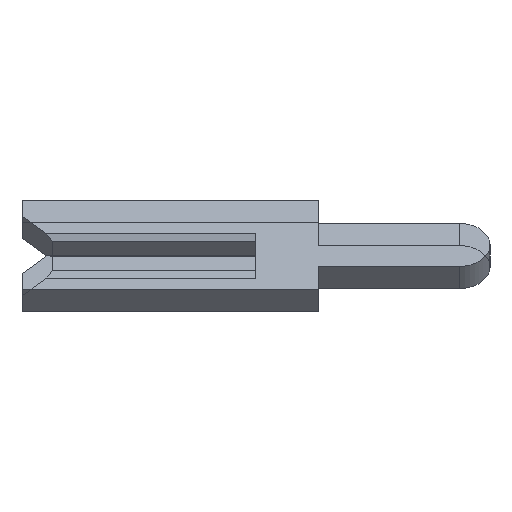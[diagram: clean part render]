
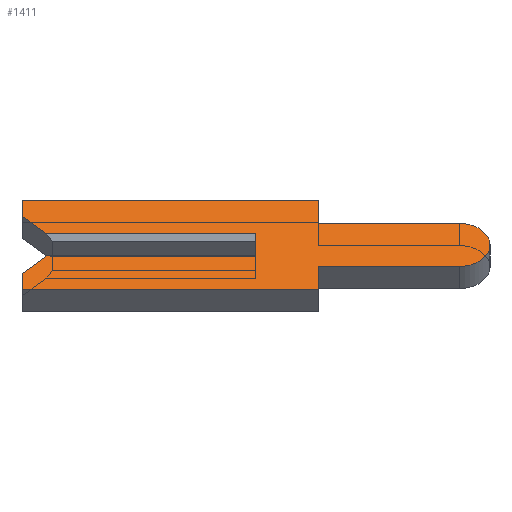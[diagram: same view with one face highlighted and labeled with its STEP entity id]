
A CAD part, left-side view. The second image highlights one B-rep face of the part: STEP entity #1411.
In plain terms, the highlighted face is planar.
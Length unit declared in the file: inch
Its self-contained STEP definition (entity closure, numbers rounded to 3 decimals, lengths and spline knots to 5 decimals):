
#4 = DIRECTION ( 'NONE',  ( 0., 0., 1. ) ) ;
#63 = VECTOR ( 'NONE', #1953, 39.37008 ) ;
#79 = VERTEX_POINT ( 'NONE', #1775 ) ;
#87 = EDGE_CURVE ( 'NONE', #1081, #1025, #403, .T. ) ;
#110 = VECTOR ( 'NONE', #1761, 39.37008 ) ;
#135 = VECTOR ( 'NONE', #1504, 39.37008 ) ;
#187 = CARTESIAN_POINT ( 'NONE',  ( -0.01, 0.1305, -0.0065 ) ) ;
#204 = VERTEX_POINT ( 'NONE', #2115 ) ;
#206 = AXIS2_PLACEMENT_3D ( 'NONE', #1594, #223, #1454 ) ;
#212 = ORIENTED_EDGE ( 'NONE', *, *, #1469, .F. ) ;
#223 = DIRECTION ( 'NONE',  ( 1., 0., 0. ) ) ;
#286 = VERTEX_POINT ( 'NONE', #1499 ) ;
#288 = CARTESIAN_POINT ( 'NONE',  ( -0.01, -0.1305, -0.01 ) ) ;
#289 = LINE ( 'NONE', #288, #135 ) ;
#359 = PLANE ( 'NONE',  #206 ) ;
#361 = VERTEX_POINT ( 'NONE', #1826 ) ;
#364 = CARTESIAN_POINT ( 'NONE',  ( -0.01, 0.15, 0.01 ) ) ;
#365 = VERTEX_POINT ( 'NONE', #1346 ) ;
#384 = CARTESIAN_POINT ( 'NONE',  ( -0.01, 0.15, 0.04 ) ) ;
#403 = LINE ( 'NONE', #755, #1865 ) ;
#416 = CARTESIAN_POINT ( 'NONE',  ( -0.01, 0.15, 0.04 ) ) ;
#417 = VERTEX_POINT ( 'NONE', #461 ) ;
#424 = LINE ( 'NONE', #416, #2146 ) ;
#461 = CARTESIAN_POINT ( 'NONE',  ( -0.01, 0.15, 0.026 ) ) ;
#474 = ORIENTED_EDGE ( 'NONE', *, *, #1277, .F. ) ;
#499 = CARTESIAN_POINT ( 'NONE',  ( -0.01, -0.04, 0.0195 ) ) ;
#509 = VECTOR ( 'NONE', #787, 39.37008 ) ;
#512 = LINE ( 'NONE', #1619, #63 ) ;
#513 = EDGE_CURVE ( 'NONE', #286, #204, #289, .T. ) ;
#547 = EDGE_CURVE ( 'NONE', #1768, #417, #993, .T. ) ;
#562 = CARTESIAN_POINT ( 'NONE',  ( -0.01, -0.04, -0.0195 ) ) ;
#570 = ORIENTED_EDGE ( 'NONE', *, *, #87, .F. ) ;
#598 = CIRCLE ( 'NONE', #1952, 0.0195 ) ;
#602 = CARTESIAN_POINT ( 'NONE',  ( -0.01, -0.04, -0.0195 ) ) ;
#607 = DIRECTION ( 'NONE',  ( 1., 0., 0. ) ) ;
#616 = LINE ( 'NONE', #1296, #2098 ) ;
#618 = DIRECTION ( 'NONE',  ( 0., 0., 1. ) ) ;
#634 = ORIENTED_EDGE ( 'NONE', *, *, #693, .F. ) ;
#638 = CARTESIAN_POINT ( 'NONE',  ( -0.01, 0.1305, 0.0065 ) ) ;
#642 = FACE_OUTER_BOUND ( 'NONE', #882, .T. ) ;
#693 = EDGE_CURVE ( 'NONE', #417, #1268, #828, .T. ) ;
#722 = LINE ( 'NONE', #187, #110 ) ;
#754 = VECTOR ( 'NONE', #1513, 39.37008 ) ;
#755 = CARTESIAN_POINT ( 'NONE',  ( -0.01, -0.04, 0.0195 ) ) ;
#776 = ORIENTED_EDGE ( 'NONE', *, *, #1968, .F. ) ;
#787 = DIRECTION ( 'NONE',  ( 0., 0., 1. ) ) ;
#802 = VECTOR ( 'NONE', #4, 39.37008 ) ;
#828 = LINE ( 'NONE', #865, #802 ) ;
#865 = CARTESIAN_POINT ( 'NONE',  ( -0.01, 0.15, 0.026 ) ) ;
#876 = VERTEX_POINT ( 'NONE', #1007 ) ;
#882 = EDGE_LOOP ( 'NONE', ( #1043, #474, #931, #1892, #2071, #776, #1511, #1441, #1754, #570, #212, #1570, #634, #1565 ) ) ;
#921 = DIRECTION ( 'NONE',  ( 0., -1., 0. ) ) ;
#931 = ORIENTED_EDGE ( 'NONE', *, *, #513, .F. ) ;
#944 = DIRECTION ( 'NONE',  ( 0., 1., 0. ) ) ;
#962 = LINE ( 'NONE', #562, #1835 ) ;
#993 = LINE ( 'NONE', #638, #754 ) ;
#1007 = CARTESIAN_POINT ( 'NONE',  ( -0.01, 0.15, -0.04 ) ) ;
#1024 = LINE ( 'NONE', #364, #1440 ) ;
#1025 = VERTEX_POINT ( 'NONE', #1061 ) ;
#1043 = ORIENTED_EDGE ( 'NONE', *, *, #1279, .T. ) ;
#1061 = CARTESIAN_POINT ( 'NONE',  ( -0.01, -0.1305, 0.0195 ) ) ;
#1081 = VERTEX_POINT ( 'NONE', #499 ) ;
#1103 = CARTESIAN_POINT ( 'NONE',  ( -0.01, 0.134, 0.01 ) ) ;
#1129 = CARTESIAN_POINT ( 'NONE',  ( -0.01, 0.15, -0.04 ) ) ;
#1246 = DIRECTION ( 'NONE',  ( 0., -1., 0. ) ) ;
#1268 = VERTEX_POINT ( 'NONE', #384 ) ;
#1277 = EDGE_CURVE ( 'NONE', #204, #365, #616, .T. ) ;
#1279 = EDGE_CURVE ( 'NONE', #1768, #365, #1024, .T. ) ;
#1296 = CARTESIAN_POINT ( 'NONE',  ( -0.01, 0., 0.0065 ) ) ;
#1318 = LINE ( 'NONE', #1974, #1352 ) ;
#1343 = EDGE_CURVE ( 'NONE', #1381, #286, #722, .T. ) ;
#1346 = CARTESIAN_POINT ( 'NONE',  ( -0.01, 0., 0.01 ) ) ;
#1352 = VECTOR ( 'NONE', #1458, 39.37008 ) ;
#1381 = VERTEX_POINT ( 'NONE', #1766 ) ;
#1397 = EDGE_CURVE ( 'NONE', #79, #1544, #962, .T. ) ;
#1411 = ADVANCED_FACE ( 'NONE', ( #642 ), #359, .F. ) ;
#1440 = VECTOR ( 'NONE', #1246, 39.37008 ) ;
#1441 = ORIENTED_EDGE ( 'NONE', *, *, #1397, .F. ) ;
#1454 = DIRECTION ( 'NONE',  ( 0., 0., -1. ) ) ;
#1458 = DIRECTION ( 'NONE',  ( 0., 0., -1. ) ) ;
#1463 = VECTOR ( 'NONE', #944, 39.37008 ) ;
#1464 = CARTESIAN_POINT ( 'NONE',  ( -0.01, -0.04, 0.04 ) ) ;
#1469 = EDGE_CURVE ( 'NONE', #1744, #1081, #512, .T. ) ;
#1499 = CARTESIAN_POINT ( 'NONE',  ( -0.01, 0.134, -0.01 ) ) ;
#1504 = DIRECTION ( 'NONE',  ( 0., -1., 0. ) ) ;
#1511 = ORIENTED_EDGE ( 'NONE', *, *, #1675, .F. ) ;
#1513 = DIRECTION ( 'NONE',  ( 0., 0.707, 0.707 ) ) ;
#1544 = VERTEX_POINT ( 'NONE', #602 ) ;
#1565 = ORIENTED_EDGE ( 'NONE', *, *, #547, .F. ) ;
#1570 = ORIENTED_EDGE ( 'NONE', *, *, #1816, .F. ) ;
#1594 = CARTESIAN_POINT ( 'NONE',  ( -0.01, -0.1305, 0. ) ) ;
#1619 = CARTESIAN_POINT ( 'NONE',  ( -0.01, -0.04, 0.04 ) ) ;
#1624 = CARTESIAN_POINT ( 'NONE',  ( -0.01, -0.1305, 0. ) ) ;
#1627 = DIRECTION ( 'NONE',  ( 0., -1., 0. ) ) ;
#1654 = LINE ( 'NONE', #2147, #509 ) ;
#1675 = EDGE_CURVE ( 'NONE', #1544, #361, #1318, .T. ) ;
#1744 = VERTEX_POINT ( 'NONE', #1464 ) ;
#1754 = ORIENTED_EDGE ( 'NONE', *, *, #1856, .F. ) ;
#1761 = DIRECTION ( 'NONE',  ( 0., -0.707, 0.707 ) ) ;
#1766 = CARTESIAN_POINT ( 'NONE',  ( -0.01, 0.15, -0.026 ) ) ;
#1768 = VERTEX_POINT ( 'NONE', #1103 ) ;
#1775 = CARTESIAN_POINT ( 'NONE',  ( -0.01, -0.1305, -0.0195 ) ) ;
#1799 = DIRECTION ( 'NONE',  ( 0., 0., -1. ) ) ;
#1816 = EDGE_CURVE ( 'NONE', #1268, #1744, #424, .T. ) ;
#1826 = CARTESIAN_POINT ( 'NONE',  ( -0.01, -0.04, -0.04 ) ) ;
#1835 = VECTOR ( 'NONE', #1940, 39.37008 ) ;
#1856 = EDGE_CURVE ( 'NONE', #1025, #79, #598, .T. ) ;
#1865 = VECTOR ( 'NONE', #1627, 39.37008 ) ;
#1892 = ORIENTED_EDGE ( 'NONE', *, *, #1343, .F. ) ;
#1940 = DIRECTION ( 'NONE',  ( 0., 1., 0. ) ) ;
#1941 = LINE ( 'NONE', #1129, #1463 ) ;
#1952 = AXIS2_PLACEMENT_3D ( 'NONE', #1624, #607, #1799 ) ;
#1953 = DIRECTION ( 'NONE',  ( 0., 0., -1. ) ) ;
#1968 = EDGE_CURVE ( 'NONE', #361, #876, #1941, .T. ) ;
#1974 = CARTESIAN_POINT ( 'NONE',  ( -0.01, -0.04, -0.04 ) ) ;
#2071 = ORIENTED_EDGE ( 'NONE', *, *, #2153, .F. ) ;
#2098 = VECTOR ( 'NONE', #618, 39.37008 ) ;
#2115 = CARTESIAN_POINT ( 'NONE',  ( -0.01, 0., -0.01 ) ) ;
#2146 = VECTOR ( 'NONE', #921, 39.37008 ) ;
#2147 = CARTESIAN_POINT ( 'NONE',  ( -0.01, 0.15, -0.026 ) ) ;
#2153 = EDGE_CURVE ( 'NONE', #876, #1381, #1654, .T. ) ;
